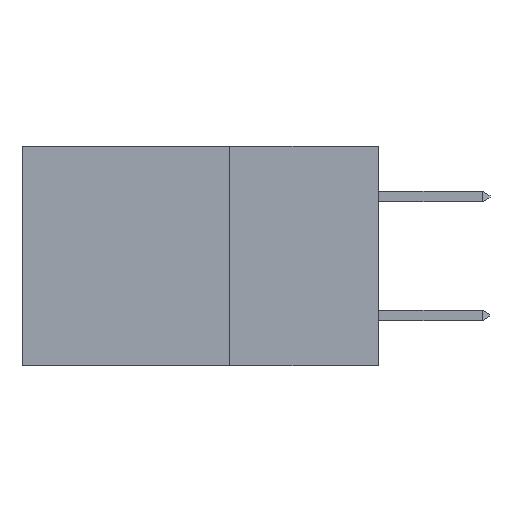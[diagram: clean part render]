
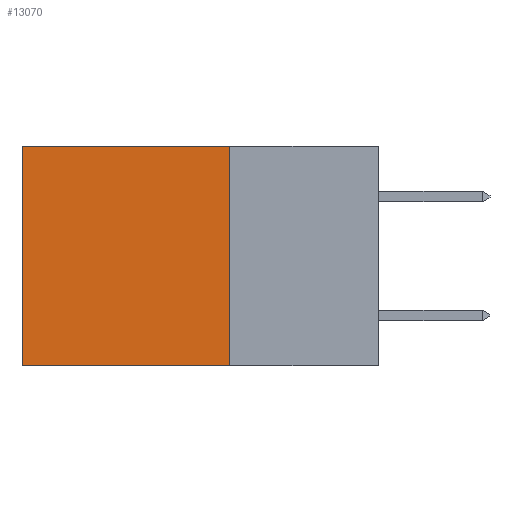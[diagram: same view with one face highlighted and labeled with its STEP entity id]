
A CAD part, left-side view. The second image highlights one B-rep face of the part: STEP entity #13070.
In plain terms, the highlighted planar face has unit normal (-1, 0, 0).
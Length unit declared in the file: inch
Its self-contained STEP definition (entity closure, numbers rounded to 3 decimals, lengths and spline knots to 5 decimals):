
#593 = DIRECTION ( 'NONE',  ( 0., 1., 0. ) ) ;
#667 = VECTOR ( 'NONE', #593, 39.37008 ) ;
#3351 = EDGE_CURVE ( 'NONE', #24424, #19665, #27676, .T. ) ;
#3717 = VERTEX_POINT ( 'NONE', #11811 ) ;
#4053 = VECTOR ( 'NONE', #19533, 39.37008 ) ;
#5471 = CARTESIAN_POINT ( 'NONE',  ( 0.298, 0.25, 0. ) ) ;
#7472 = EDGE_CURVE ( 'NONE', #3717, #19665, #13801, .T. ) ;
#8514 = ORIENTED_EDGE ( 'NONE', *, *, #26909, .T. ) ;
#8892 = CARTESIAN_POINT ( 'NONE',  ( 0.298, 0.25, 0. ) ) ;
#9345 = CARTESIAN_POINT ( 'NONE',  ( 0.298, 0.25, 0. ) ) ;
#10997 = CARTESIAN_POINT ( 'NONE',  ( 0.298, 0.6, 0. ) ) ;
#11065 = EDGE_LOOP ( 'NONE', ( #17767, #25283, #26755, #8514 ) ) ;
#11264 = LINE ( 'NONE', #9345, #23159 ) ;
#11581 = DIRECTION ( 'NONE',  ( 0., 0., -1. ) ) ;
#11811 = CARTESIAN_POINT ( 'NONE',  ( 0.298, 0.25, -0.37 ) ) ;
#12400 = VECTOR ( 'NONE', #18719, 39.37008 ) ;
#13070 = ADVANCED_FACE ( 'NONE', ( #21909 ), #25504, .F. ) ;
#13801 = LINE ( 'NONE', #22720, #667 ) ;
#14384 = DIRECTION ( 'NONE',  ( 0., 0., -1. ) ) ;
#15054 = CARTESIAN_POINT ( 'NONE',  ( 0.298, 0.6, 0. ) ) ;
#16006 = CARTESIAN_POINT ( 'NONE',  ( 0.298, 0.6, -0.37 ) ) ;
#16541 = CARTESIAN_POINT ( 'NONE',  ( 0.298, 0.25, 0. ) ) ;
#17767 = ORIENTED_EDGE ( 'NONE', *, *, #3351, .T. ) ;
#18719 = DIRECTION ( 'NONE',  ( 0., 1., 0. ) ) ;
#19533 = DIRECTION ( 'NONE',  ( 0., 0., -1. ) ) ;
#19665 = VERTEX_POINT ( 'NONE', #16006 ) ;
#21909 = FACE_OUTER_BOUND ( 'NONE', #11065, .T. ) ;
#22658 = EDGE_CURVE ( 'NONE', #26745, #3717, #11264, .T. ) ;
#22720 = CARTESIAN_POINT ( 'NONE',  ( 0.298, 0.25, -0.37 ) ) ;
#23159 = VECTOR ( 'NONE', #11581, 39.37008 ) ;
#23578 = LINE ( 'NONE', #5471, #12400 ) ;
#24424 = VERTEX_POINT ( 'NONE', #10997 ) ;
#24562 = AXIS2_PLACEMENT_3D ( 'NONE', #16541, #27731, #14384 ) ;
#25283 = ORIENTED_EDGE ( 'NONE', *, *, #7472, .F. ) ;
#25504 = PLANE ( 'NONE',  #24562 ) ;
#26745 = VERTEX_POINT ( 'NONE', #8892 ) ;
#26755 = ORIENTED_EDGE ( 'NONE', *, *, #22658, .F. ) ;
#26909 = EDGE_CURVE ( 'NONE', #26745, #24424, #23578, .T. ) ;
#27676 = LINE ( 'NONE', #15054, #4053 ) ;
#27731 = DIRECTION ( 'NONE',  ( 1., 0., 0. ) ) ;
